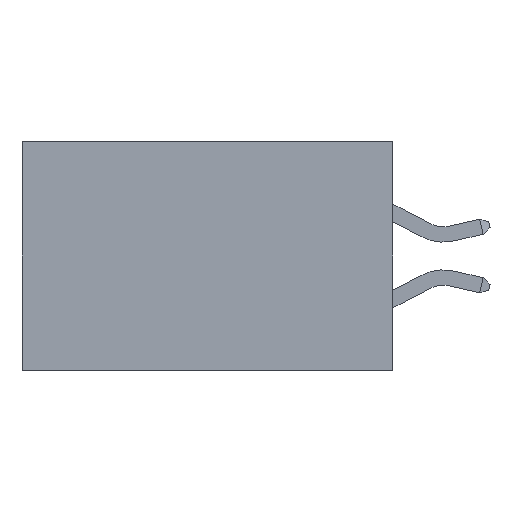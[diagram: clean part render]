
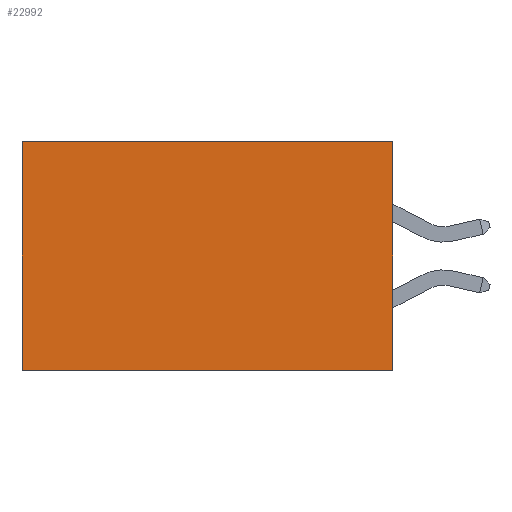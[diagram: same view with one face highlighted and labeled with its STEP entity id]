
A CAD part, left-side view. The second image highlights one B-rep face of the part: STEP entity #22992.
In plain terms, the highlighted planar face has unit normal (-1, 0, 0).
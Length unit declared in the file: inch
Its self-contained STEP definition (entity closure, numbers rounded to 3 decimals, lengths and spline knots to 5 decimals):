
#18 = LINE ( 'NONE', #22040, #23080 ) ;
#648 = VERTEX_POINT ( 'NONE', #4891 ) ;
#1586 = EDGE_LOOP ( 'NONE', ( #19596, #3662, #12115, #24083 ) ) ;
#1672 = AXIS2_PLACEMENT_3D ( 'NONE', #17957, #9484, #22239 ) ;
#3662 = ORIENTED_EDGE ( 'NONE', *, *, #7193, .F. ) ;
#4891 = CARTESIAN_POINT ( 'NONE',  ( 0.2875, 0.6, 0. ) ) ;
#6081 = VERTEX_POINT ( 'NONE', #14860 ) ;
#6469 = DIRECTION ( 'NONE',  ( 0., 0., -1. ) ) ;
#6734 = FACE_OUTER_BOUND ( 'NONE', #1586, .T. ) ;
#7112 = CARTESIAN_POINT ( 'NONE',  ( 0.2875, 0., -0.37 ) ) ;
#7193 = EDGE_CURVE ( 'NONE', #24232, #21297, #18, .T. ) ;
#9484 = DIRECTION ( 'NONE',  ( 1., 0., 0. ) ) ;
#11228 = DIRECTION ( 'NONE',  ( 0., 1., 0. ) ) ;
#12115 = ORIENTED_EDGE ( 'NONE', *, *, #17584, .F. ) ;
#12502 = LINE ( 'NONE', #21447, #16832 ) ;
#13107 = LINE ( 'NONE', #21604, #24470 ) ;
#14696 = EDGE_CURVE ( 'NONE', #648, #21297, #16551, .T. ) ;
#14860 = CARTESIAN_POINT ( 'NONE',  ( 0.2875, 0., 0. ) ) ;
#16551 = LINE ( 'NONE', #22931, #18551 ) ;
#16812 = EDGE_CURVE ( 'NONE', #6081, #648, #12502, .T. ) ;
#16832 = VECTOR ( 'NONE', #27702, 39.37008 ) ;
#17584 = EDGE_CURVE ( 'NONE', #6081, #24232, #13107, .T. ) ;
#17953 = CARTESIAN_POINT ( 'NONE',  ( 0.2875, 0.6, -0.37 ) ) ;
#17957 = CARTESIAN_POINT ( 'NONE',  ( 0.2875, 0., 0. ) ) ;
#18551 = VECTOR ( 'NONE', #27293, 39.37008 ) ;
#19596 = ORIENTED_EDGE ( 'NONE', *, *, #14696, .T. ) ;
#21297 = VERTEX_POINT ( 'NONE', #17953 ) ;
#21447 = CARTESIAN_POINT ( 'NONE',  ( 0.2875, 0., 0. ) ) ;
#21604 = CARTESIAN_POINT ( 'NONE',  ( 0.2875, 0., 0. ) ) ;
#22040 = CARTESIAN_POINT ( 'NONE',  ( 0.2875, 0., -0.37 ) ) ;
#22239 = DIRECTION ( 'NONE',  ( 0., 0., -1. ) ) ;
#22931 = CARTESIAN_POINT ( 'NONE',  ( 0.2875, 0.6, 0. ) ) ;
#22992 = ADVANCED_FACE ( 'NONE', ( #6734 ), #26389, .F. ) ;
#23080 = VECTOR ( 'NONE', #11228, 39.37008 ) ;
#24083 = ORIENTED_EDGE ( 'NONE', *, *, #16812, .T. ) ;
#24232 = VERTEX_POINT ( 'NONE', #7112 ) ;
#24470 = VECTOR ( 'NONE', #6469, 39.37008 ) ;
#26389 = PLANE ( 'NONE',  #1672 ) ;
#27293 = DIRECTION ( 'NONE',  ( 0., 0., -1. ) ) ;
#27702 = DIRECTION ( 'NONE',  ( 0., 1., 0. ) ) ;
